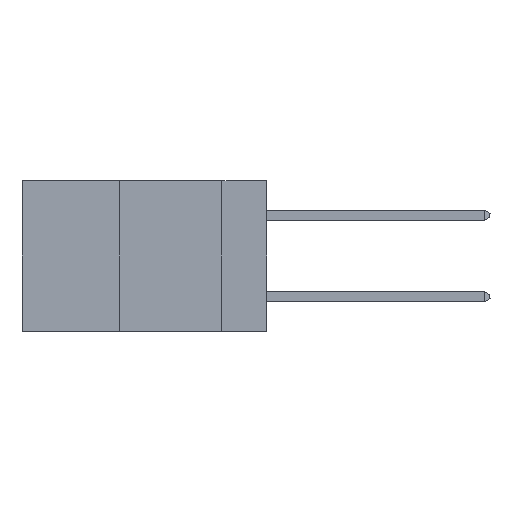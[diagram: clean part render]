
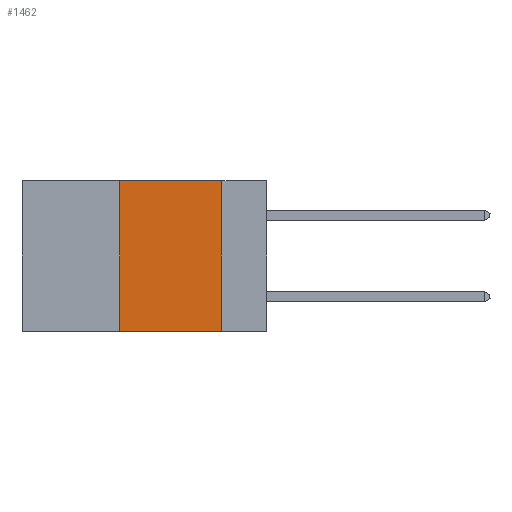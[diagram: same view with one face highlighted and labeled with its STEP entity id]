
A CAD part, left-side view. The second image highlights one B-rep face of the part: STEP entity #1462.
In plain terms, the highlighted planar face has unit normal (-1, 0, 0).
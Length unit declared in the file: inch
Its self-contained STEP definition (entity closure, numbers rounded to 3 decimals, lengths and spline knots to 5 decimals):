
#100 = CARTESIAN_POINT ( 'NONE',  ( 0., 0.36, 0. ) ) ;
#1462 = ADVANCED_FACE ( 'NONE', ( #11675 ), #9595, .F. ) ;
#3234 = DIRECTION ( 'NONE',  ( 0., 0., 1. ) ) ;
#3833 = DIRECTION ( 'NONE',  ( 0., 0., -1. ) ) ;
#4742 = LINE ( 'NONE', #100, #20346 ) ;
#6037 = EDGE_LOOP ( 'NONE', ( #27317, #33991, #32244, #29775 ) ) ;
#6597 = AXIS2_PLACEMENT_3D ( 'NONE', #25266, #31215, #15747 ) ;
#7716 = DIRECTION ( 'NONE',  ( 0., -1., 0. ) ) ;
#8108 = VERTEX_POINT ( 'NONE', #18729 ) ;
#8236 = CARTESIAN_POINT ( 'NONE',  ( 0., 0.6, -0.37 ) ) ;
#9572 = VERTEX_POINT ( 'NONE', #18179 ) ;
#9595 = PLANE ( 'NONE',  #6597 ) ;
#10737 = CARTESIAN_POINT ( 'NONE',  ( 0., 0.6, 0. ) ) ;
#10905 = VERTEX_POINT ( 'NONE', #14832 ) ;
#11544 = DIRECTION ( 'NONE',  ( 0., -1., 0. ) ) ;
#11675 = FACE_OUTER_BOUND ( 'NONE', #6037, .T. ) ;
#13120 = VERTEX_POINT ( 'NONE', #34519 ) ;
#14526 = EDGE_CURVE ( 'NONE', #8108, #13120, #18871, .T. ) ;
#14832 = CARTESIAN_POINT ( 'NONE',  ( 0., 0.36, -0.37 ) ) ;
#15747 = DIRECTION ( 'NONE',  ( 0., 0., -1. ) ) ;
#18179 = CARTESIAN_POINT ( 'NONE',  ( 0., 0.36, 0. ) ) ;
#18729 = CARTESIAN_POINT ( 'NONE',  ( 0., 0.11, 0. ) ) ;
#18871 = LINE ( 'NONE', #22906, #21311 ) ;
#20346 = VECTOR ( 'NONE', #3234, 39.37008 ) ;
#20487 = LINE ( 'NONE', #8236, #36959 ) ;
#20515 = VECTOR ( 'NONE', #7716, 39.37008 ) ;
#21311 = VECTOR ( 'NONE', #3833, 39.37008 ) ;
#22215 = EDGE_CURVE ( 'NONE', #9572, #8108, #32153, .T. ) ;
#22906 = CARTESIAN_POINT ( 'NONE',  ( 0., 0.11, 0. ) ) ;
#25266 = CARTESIAN_POINT ( 'NONE',  ( 0., 0.6, 0. ) ) ;
#27317 = ORIENTED_EDGE ( 'NONE', *, *, #14526, .F. ) ;
#29775 = ORIENTED_EDGE ( 'NONE', *, *, #38342, .T. ) ;
#30737 = EDGE_CURVE ( 'NONE', #10905, #9572, #4742, .T. ) ;
#31215 = DIRECTION ( 'NONE',  ( 1., 0., 0. ) ) ;
#32153 = LINE ( 'NONE', #10737, #20515 ) ;
#32244 = ORIENTED_EDGE ( 'NONE', *, *, #30737, .F. ) ;
#33991 = ORIENTED_EDGE ( 'NONE', *, *, #22215, .F. ) ;
#34519 = CARTESIAN_POINT ( 'NONE',  ( 0., 0.11, -0.37 ) ) ;
#36959 = VECTOR ( 'NONE', #11544, 39.37008 ) ;
#38342 = EDGE_CURVE ( 'NONE', #10905, #13120, #20487, .T. ) ;
